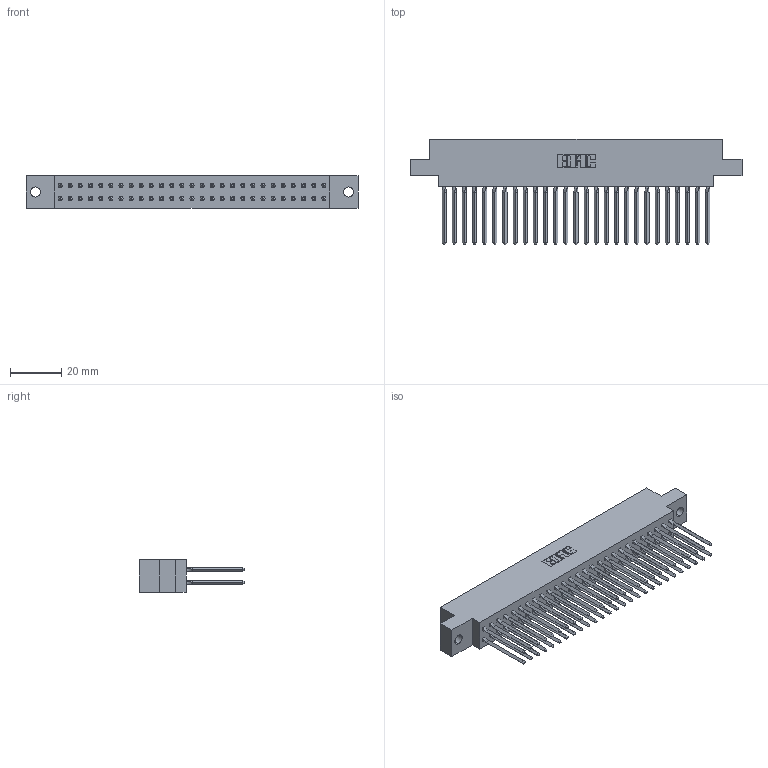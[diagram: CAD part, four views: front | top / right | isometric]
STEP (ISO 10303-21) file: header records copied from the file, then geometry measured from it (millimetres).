
FILE_DESCRIPTION (( 'STEP AP203' ), '1' );
FILE_NAME ('317-054-543-804.STEP', '2020-02-28T04:04:46', ( '' ), ( '' ), 'SwSTEP 2.0', 'SolidWorks 2016', '' );
FILE_SCHEMA (( 'CONFIG_CONTROL_DESIGN' ));
Length unit declared in the file: inch
Products named in the file (3): 317-054-543-804; 317-290-001_543; 317 Part_.156 Dia - TH
Assembly tree (55 placements, depth 2):
  317-054-543-804
    317 Part_.156 Dia - TH
    317-290-001_543  x54
Bounding box: 129.69 x 41.15 x 12.7 mm (x, y, z)
Volume: 21440.1 mm3; surface area: 31763.7 mm2
Topology: 55 solids, 55 shells, 4908 faces, 13613 edges, 8768 vertices
Faces by surface type: plane 4000, cylinder 692, bspline 216
Entity records: 41124 total; most frequent: CARTESIAN_POINT 7587, ORIENTED_EDGE 7086, DIRECTION 5913, EDGE_CURVE 3543, LINE 3287, VECTOR 3287, VERTEX_POINT 2355, AXIS2_PLACEMENT_3D 1313
